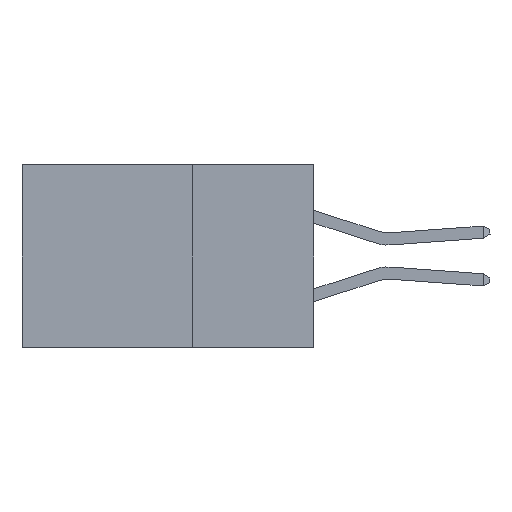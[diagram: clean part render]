
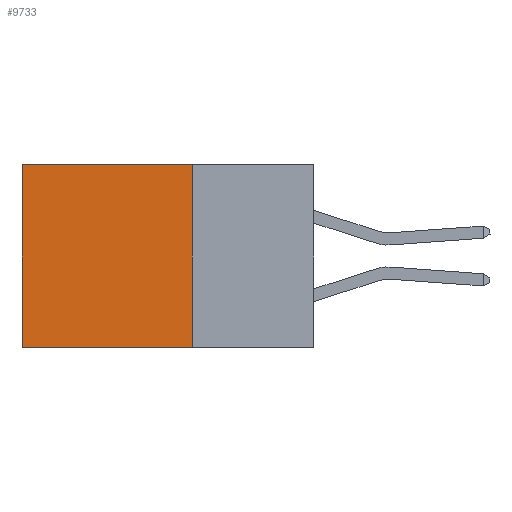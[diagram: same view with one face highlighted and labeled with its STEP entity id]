
A CAD part, left-side view. The second image highlights one B-rep face of the part: STEP entity #9733.
In plain terms, the highlighted planar face has unit normal (-1, 0, 0).
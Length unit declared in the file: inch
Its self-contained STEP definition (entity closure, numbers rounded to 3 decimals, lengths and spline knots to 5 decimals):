
#644 = CARTESIAN_POINT ( 'NONE',  ( 0.2875, 0.6, -0.375 ) ) ;
#873 = EDGE_LOOP ( 'NONE', ( #2391, #4587, #1266, #7191 ) ) ;
#1266 = ORIENTED_EDGE ( 'NONE', *, *, #8144, .F. ) ;
#1521 = CARTESIAN_POINT ( 'NONE',  ( 0.2875, 0.25, -0.375 ) ) ;
#1573 = LINE ( 'NONE', #4538, #7368 ) ;
#1628 = EDGE_CURVE ( 'NONE', #5504, #8513, #8537, .T. ) ;
#1949 = VERTEX_POINT ( 'NONE', #4103 ) ;
#2188 = EDGE_CURVE ( 'NONE', #8572, #8513, #5817, .T. ) ;
#2388 = CARTESIAN_POINT ( 'NONE',  ( 0.2875, 0.6, 0. ) ) ;
#2391 = ORIENTED_EDGE ( 'NONE', *, *, #1628, .T. ) ;
#2559 = DIRECTION ( 'NONE',  ( 0., 0., -1. ) ) ;
#3071 = VECTOR ( 'NONE', #6106, 39.37008 ) ;
#4103 = CARTESIAN_POINT ( 'NONE',  ( 0.2875, 0.25, 0. ) ) ;
#4268 = EDGE_CURVE ( 'NONE', #1949, #5504, #1573, .T. ) ;
#4538 = CARTESIAN_POINT ( 'NONE',  ( 0.2875, 0.25, 0. ) ) ;
#4587 = ORIENTED_EDGE ( 'NONE', *, *, #2188, .F. ) ;
#5173 = DIRECTION ( 'NONE',  ( 0., 0., -1. ) ) ;
#5296 = DIRECTION ( 'NONE',  ( 0., 1., 0. ) ) ;
#5504 = VERTEX_POINT ( 'NONE', #2388 ) ;
#5817 = LINE ( 'NONE', #1521, #3071 ) ;
#5879 = VECTOR ( 'NONE', #2559, 39.37008 ) ;
#6106 = DIRECTION ( 'NONE',  ( 0., 1., 0. ) ) ;
#6419 = CARTESIAN_POINT ( 'NONE',  ( 0.2875, 0.25, -0.375 ) ) ;
#6630 = CARTESIAN_POINT ( 'NONE',  ( 0.2875, 0.25, -0.375 ) ) ;
#7097 = AXIS2_PLACEMENT_3D ( 'NONE', #6630, #7354, #8860 ) ;
#7191 = ORIENTED_EDGE ( 'NONE', *, *, #4268, .T. ) ;
#7327 = PLANE ( 'NONE',  #7097 ) ;
#7354 = DIRECTION ( 'NONE',  ( 1., 0., 0. ) ) ;
#7368 = VECTOR ( 'NONE', #5296, 39.37008 ) ;
#8144 = EDGE_CURVE ( 'NONE', #1949, #8572, #9413, .T. ) ;
#8214 = FACE_OUTER_BOUND ( 'NONE', #873, .T. ) ;
#8513 = VERTEX_POINT ( 'NONE', #644 ) ;
#8537 = LINE ( 'NONE', #9565, #9243 ) ;
#8572 = VERTEX_POINT ( 'NONE', #9722 ) ;
#8860 = DIRECTION ( 'NONE',  ( 0., 0., -1. ) ) ;
#9243 = VECTOR ( 'NONE', #5173, 39.37008 ) ;
#9413 = LINE ( 'NONE', #6419, #5879 ) ;
#9565 = CARTESIAN_POINT ( 'NONE',  ( 0.2875, 0.6, -0.375 ) ) ;
#9722 = CARTESIAN_POINT ( 'NONE',  ( 0.2875, 0.25, -0.375 ) ) ;
#9733 = ADVANCED_FACE ( 'NONE', ( #8214 ), #7327, .F. ) ;
